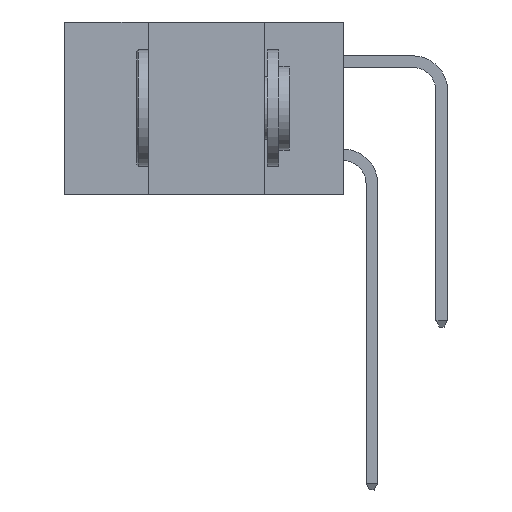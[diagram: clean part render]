
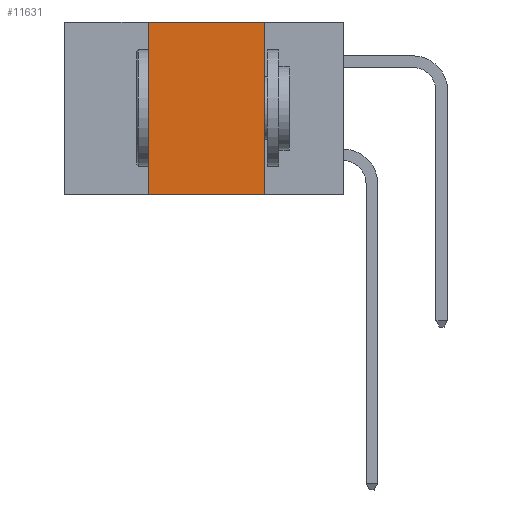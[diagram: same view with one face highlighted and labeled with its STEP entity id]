
A CAD part, left-side view. The second image highlights one B-rep face of the part: STEP entity #11631.
In plain terms, the highlighted planar face has unit normal (-1, 0, 0).
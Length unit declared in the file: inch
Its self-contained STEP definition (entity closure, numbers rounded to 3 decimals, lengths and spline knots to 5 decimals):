
#138 = ORIENTED_EDGE ( 'NONE', *, *, #9799, .T. ) ;
#815 = LINE ( 'NONE', #2287, #14547 ) ;
#823 = DIRECTION ( 'NONE',  ( 0., 0., 1. ) ) ;
#825 = CARTESIAN_POINT ( 'NONE',  ( 0., 0.17, -0.37 ) ) ;
#1137 = CARTESIAN_POINT ( 'NONE',  ( 0., 0.6, -0.37 ) ) ;
#1145 = VERTEX_POINT ( 'NONE', #15918 ) ;
#2076 = ORIENTED_EDGE ( 'NONE', *, *, #13781, .F. ) ;
#2238 = VERTEX_POINT ( 'NONE', #8592 ) ;
#2287 = CARTESIAN_POINT ( 'NONE',  ( 0., 0.42, 0. ) ) ;
#2385 = DIRECTION ( 'NONE',  ( 0., 0., -1. ) ) ;
#2505 = ORIENTED_EDGE ( 'NONE', *, *, #8917, .F. ) ;
#2843 = DIRECTION ( 'NONE',  ( 0., -1., 0. ) ) ;
#3512 = VECTOR ( 'NONE', #2385, 39.37008 ) ;
#3966 = VERTEX_POINT ( 'NONE', #5851 ) ;
#4700 = LINE ( 'NONE', #10918, #5305 ) ;
#5305 = VECTOR ( 'NONE', #2843, 39.37008 ) ;
#5851 = CARTESIAN_POINT ( 'NONE',  ( 0., 0.42, 0. ) ) ;
#7100 = ORIENTED_EDGE ( 'NONE', *, *, #8042, .F. ) ;
#7180 = LINE ( 'NONE', #14213, #3512 ) ;
#7757 = DIRECTION ( 'NONE',  ( 0., 0., -1. ) ) ;
#8042 = EDGE_CURVE ( 'NONE', #2238, #15424, #7180, .T. ) ;
#8437 = VECTOR ( 'NONE', #15694, 39.37008 ) ;
#8592 = CARTESIAN_POINT ( 'NONE',  ( 0., 0.17, 0. ) ) ;
#8917 = EDGE_CURVE ( 'NONE', #1145, #3966, #815, .T. ) ;
#9029 = CARTESIAN_POINT ( 'NONE',  ( 0., 0.6, 0. ) ) ;
#9799 = EDGE_CURVE ( 'NONE', #1145, #15424, #11858, .T. ) ;
#9988 = EDGE_LOOP ( 'NONE', ( #7100, #2076, #2505, #138 ) ) ;
#10431 = FACE_OUTER_BOUND ( 'NONE', #9988, .T. ) ;
#10918 = CARTESIAN_POINT ( 'NONE',  ( 0., 0.6, 0. ) ) ;
#11609 = PLANE ( 'NONE',  #13709 ) ;
#11631 = ADVANCED_FACE ( 'NONE', ( #10431 ), #11609, .F. ) ;
#11858 = LINE ( 'NONE', #1137, #8437 ) ;
#13709 = AXIS2_PLACEMENT_3D ( 'NONE', #9029, #15318, #7757 ) ;
#13781 = EDGE_CURVE ( 'NONE', #3966, #2238, #4700, .T. ) ;
#14213 = CARTESIAN_POINT ( 'NONE',  ( 0., 0.17, 0. ) ) ;
#14547 = VECTOR ( 'NONE', #823, 39.37008 ) ;
#15318 = DIRECTION ( 'NONE',  ( 1., 0., 0. ) ) ;
#15424 = VERTEX_POINT ( 'NONE', #825 ) ;
#15694 = DIRECTION ( 'NONE',  ( 0., -1., 0. ) ) ;
#15918 = CARTESIAN_POINT ( 'NONE',  ( 0., 0.42, -0.37 ) ) ;
